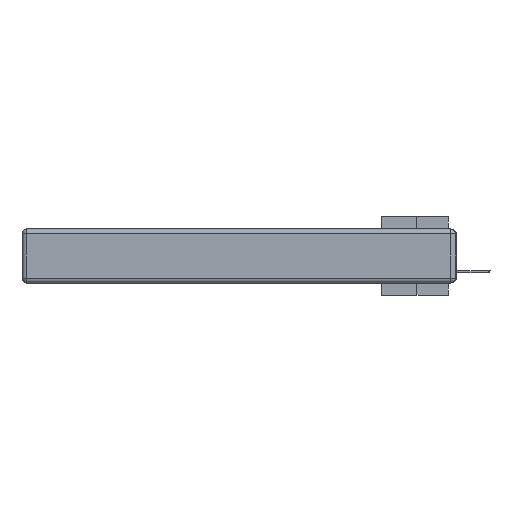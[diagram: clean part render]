
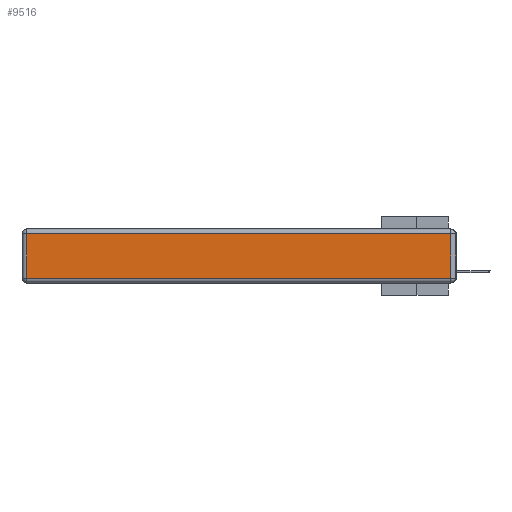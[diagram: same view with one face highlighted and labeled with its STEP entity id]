
A CAD part, left-side view. The second image highlights one B-rep face of the part: STEP entity #9516.
In plain terms, the highlighted planar face has unit normal (-1, 0, 0).
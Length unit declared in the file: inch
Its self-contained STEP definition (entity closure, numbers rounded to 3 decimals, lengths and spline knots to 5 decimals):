
#1535 = DIRECTION ( 'NONE',  ( 0., -1., 0. ) ) ;
#1759 = LINE ( 'NONE', #28668, #19743 ) ;
#2779 = CARTESIAN_POINT ( 'NONE',  ( 0., 2.72, -0.313 ) ) ;
#2805 = FACE_OUTER_BOUND ( 'NONE', #3289, .T. ) ;
#2838 = CARTESIAN_POINT ( 'NONE',  ( 0., 0.03, -0.313 ) ) ;
#3289 = EDGE_LOOP ( 'NONE', ( #11750, #26352, #17369, #9064 ) ) ;
#4410 = VERTEX_POINT ( 'NONE', #7696 ) ;
#4581 = DIRECTION ( 'NONE',  ( 0., 0., 1. ) ) ;
#6964 = CARTESIAN_POINT ( 'NONE',  ( 0., 2.75, -0.03 ) ) ;
#7696 = CARTESIAN_POINT ( 'NONE',  ( 0., 2.72, -0.03 ) ) ;
#8143 = EDGE_CURVE ( 'NONE', #27052, #25237, #33334, .T. ) ;
#8835 = VECTOR ( 'NONE', #12197, 39.37008 ) ;
#8947 = DIRECTION ( 'NONE',  ( 0., 0., -1. ) ) ;
#9064 = ORIENTED_EDGE ( 'NONE', *, *, #20525, .T. ) ;
#9516 = ADVANCED_FACE ( 'NONE', ( #2805 ), #18287, .T. ) ;
#11750 = ORIENTED_EDGE ( 'NONE', *, *, #8143, .T. ) ;
#12197 = DIRECTION ( 'NONE',  ( 0., 1., 0. ) ) ;
#13491 = CARTESIAN_POINT ( 'NONE',  ( 0., 0.03, -0.03 ) ) ;
#13786 = VERTEX_POINT ( 'NONE', #13491 ) ;
#14641 = EDGE_CURVE ( 'NONE', #25237, #13786, #1759, .T. ) ;
#15018 = DIRECTION ( 'NONE',  ( 0., 0., 1. ) ) ;
#17369 = ORIENTED_EDGE ( 'NONE', *, *, #19146, .T. ) ;
#18065 = CARTESIAN_POINT ( 'NONE',  ( 0., 0., -0.313 ) ) ;
#18287 = PLANE ( 'NONE',  #24927 ) ;
#19146 = EDGE_CURVE ( 'NONE', #13786, #4410, #31732, .T. ) ;
#19743 = VECTOR ( 'NONE', #15018, 39.37008 ) ;
#20525 = EDGE_CURVE ( 'NONE', #4410, #27052, #29606, .T. ) ;
#23475 = DIRECTION ( 'NONE',  ( -1., 0., 0. ) ) ;
#23734 = CARTESIAN_POINT ( 'NONE',  ( 0., 0., -0.343 ) ) ;
#24927 = AXIS2_PLACEMENT_3D ( 'NONE', #23734, #23475, #4581 ) ;
#25237 = VERTEX_POINT ( 'NONE', #2838 ) ;
#26352 = ORIENTED_EDGE ( 'NONE', *, *, #14641, .T. ) ;
#27052 = VERTEX_POINT ( 'NONE', #2779 ) ;
#28668 = CARTESIAN_POINT ( 'NONE',  ( 0., 0.03, -0.343 ) ) ;
#29606 = LINE ( 'NONE', #31273, #32616 ) ;
#30325 = VECTOR ( 'NONE', #1535, 39.37008 ) ;
#31273 = CARTESIAN_POINT ( 'NONE',  ( 0., 2.72, -0.343 ) ) ;
#31732 = LINE ( 'NONE', #6964, #8835 ) ;
#32616 = VECTOR ( 'NONE', #8947, 39.37008 ) ;
#33334 = LINE ( 'NONE', #18065, #30325 ) ;
